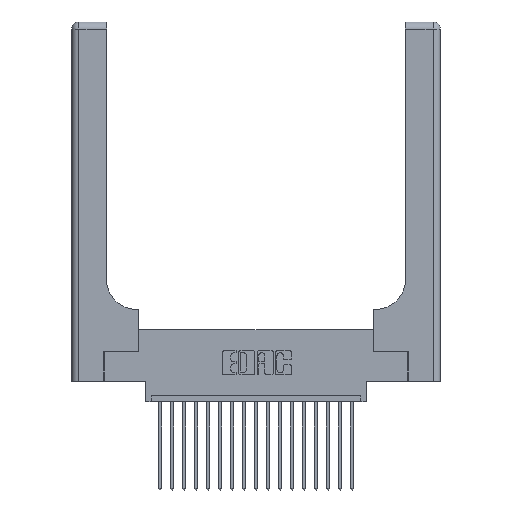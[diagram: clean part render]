
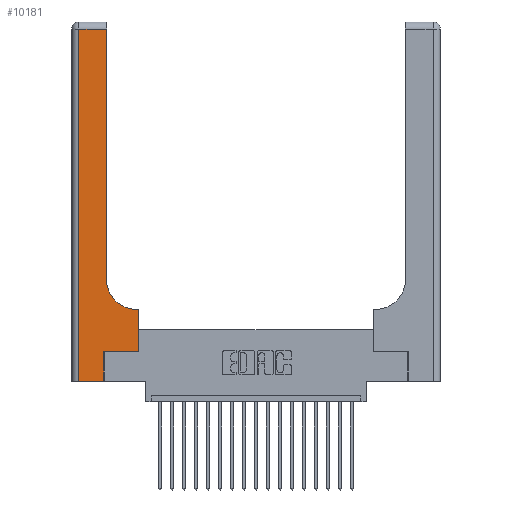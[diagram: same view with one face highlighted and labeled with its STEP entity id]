
A CAD part, top view. The second image highlights one B-rep face of the part: STEP entity #10181.
In plain terms, the highlighted planar face has unit normal (0, 0, 1).
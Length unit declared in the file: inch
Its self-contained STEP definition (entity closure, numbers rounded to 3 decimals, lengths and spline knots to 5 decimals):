
#115 = EDGE_CURVE ( 'NONE', #12358, #16170, #7274, .T. ) ;
#128 = CIRCLE ( 'NONE', #13776, 0.25 ) ;
#336 = ORIENTED_EDGE ( 'NONE', *, *, #13249, .T. ) ;
#466 = DIRECTION ( 'NONE',  ( -1., 0., 0. ) ) ;
#657 = ORIENTED_EDGE ( 'NONE', *, *, #16451, .T. ) ;
#726 = CARTESIAN_POINT ( 'NONE',  ( 0., 2.94, 0.37 ) ) ;
#1083 = CARTESIAN_POINT ( 'NONE',  ( 0.5585, 0.6, 0.37 ) ) ;
#1339 = VECTOR ( 'NONE', #5027, 39.37008 ) ;
#1526 = VERTEX_POINT ( 'NONE', #1083 ) ;
#1800 = VERTEX_POINT ( 'NONE', #20786 ) ;
#1990 = LINE ( 'NONE', #4769, #4318 ) ;
#2366 = DIRECTION ( 'NONE',  ( -1., 0., 0. ) ) ;
#2851 = ORIENTED_EDGE ( 'NONE', *, *, #115, .T. ) ;
#2908 = LINE ( 'NONE', #726, #19296 ) ;
#3039 = CARTESIAN_POINT ( 'NONE',  ( 0.2915, 3., 0.37 ) ) ;
#3593 = EDGE_CURVE ( 'NONE', #18591, #9116, #13647, .T. ) ;
#3760 = EDGE_CURVE ( 'NONE', #1800, #12052, #10984, .T. ) ;
#4318 = VECTOR ( 'NONE', #21324, 39.37008 ) ;
#4769 = CARTESIAN_POINT ( 'NONE',  ( 0.5585, 0.25, 0.37 ) ) ;
#4877 = CARTESIAN_POINT ( 'NONE',  ( 0.269, 0., 0.37 ) ) ;
#5027 = DIRECTION ( 'NONE',  ( 0., 1., 0. ) ) ;
#5097 = EDGE_CURVE ( 'NONE', #13422, #18591, #128, .T. ) ;
#5356 = VECTOR ( 'NONE', #19885, 39.37008 ) ;
#5435 = CARTESIAN_POINT ( 'NONE',  ( 0.269, 0.25, 0.37 ) ) ;
#5664 = DIRECTION ( 'NONE',  ( -1., 0., 0. ) ) ;
#6157 = CARTESIAN_POINT ( 'NONE',  ( 0.269, 0., 0.37 ) ) ;
#6214 = FACE_OUTER_BOUND ( 'NONE', #17953, .T. ) ;
#6238 = VECTOR ( 'NONE', #6935, 39.37008 ) ;
#6370 = DIRECTION ( 'NONE',  ( 0., 0., -1. ) ) ;
#6437 = VECTOR ( 'NONE', #19511, 39.37008 ) ;
#6935 = DIRECTION ( 'NONE',  ( 1., 0., 0. ) ) ;
#7274 = LINE ( 'NONE', #5435, #6238 ) ;
#7330 = ORIENTED_EDGE ( 'NONE', *, *, #13846, .T. ) ;
#7366 = CARTESIAN_POINT ( 'NONE',  ( 0.5415, 0.6, 0.37 ) ) ;
#7456 = AXIS2_PLACEMENT_3D ( 'NONE', #8731, #13614, #466 ) ;
#7781 = LINE ( 'NONE', #4877, #1339 ) ;
#8046 = CARTESIAN_POINT ( 'NONE',  ( 0.5585, 0.25, 0.37 ) ) ;
#8447 = ORIENTED_EDGE ( 'NONE', *, *, #5097, .T. ) ;
#8731 = CARTESIAN_POINT ( 'NONE',  ( 0., 3., 0.37 ) ) ;
#9116 = VERTEX_POINT ( 'NONE', #10461 ) ;
#10181 = ADVANCED_FACE ( 'NONE', ( #6214 ), #18722, .F. ) ;
#10461 = CARTESIAN_POINT ( 'NONE',  ( 0.2915, 2.94, 0.37 ) ) ;
#10879 = EDGE_CURVE ( 'NONE', #13463, #1800, #18939, .T. ) ;
#10984 = LINE ( 'NONE', #21500, #5356 ) ;
#11187 = DIRECTION ( 'NONE',  ( 0., 1., 0. ) ) ;
#11348 = DIRECTION ( 'NONE',  ( 1., 0., 0. ) ) ;
#11429 = CARTESIAN_POINT ( 'NONE',  ( 0.5415, 0.85, 0.37 ) ) ;
#12052 = VERTEX_POINT ( 'NONE', #6157 ) ;
#12358 = VERTEX_POINT ( 'NONE', #21292 ) ;
#13249 = EDGE_CURVE ( 'NONE', #1526, #13422, #17293, .T. ) ;
#13422 = VERTEX_POINT ( 'NONE', #7366 ) ;
#13463 = VERTEX_POINT ( 'NONE', #19082 ) ;
#13592 = ORIENTED_EDGE ( 'NONE', *, *, #3593, .T. ) ;
#13614 = DIRECTION ( 'NONE',  ( 0., 0., -1. ) ) ;
#13647 = LINE ( 'NONE', #3039, #17283 ) ;
#13776 = AXIS2_PLACEMENT_3D ( 'NONE', #11429, #6370, #11348 ) ;
#13846 = EDGE_CURVE ( 'NONE', #16170, #1526, #1990, .T. ) ;
#14249 = ORIENTED_EDGE ( 'NONE', *, *, #10879, .T. ) ;
#16170 = VERTEX_POINT ( 'NONE', #8046 ) ;
#16451 = EDGE_CURVE ( 'NONE', #9116, #13463, #2908, .T. ) ;
#16795 = ORIENTED_EDGE ( 'NONE', *, *, #3760, .T. ) ;
#17084 = CARTESIAN_POINT ( 'NONE',  ( 0.2915, 0.85, 0.37 ) ) ;
#17283 = VECTOR ( 'NONE', #11187, 39.37008 ) ;
#17293 = LINE ( 'NONE', #19020, #17811 ) ;
#17518 = EDGE_CURVE ( 'NONE', #12052, #12358, #7781, .T. ) ;
#17811 = VECTOR ( 'NONE', #5664, 39.37008 ) ;
#17953 = EDGE_LOOP ( 'NONE', ( #13592, #657, #14249, #16795, #19897, #2851, #7330, #336, #8447 ) ) ;
#18591 = VERTEX_POINT ( 'NONE', #17084 ) ;
#18722 = PLANE ( 'NONE',  #7456 ) ;
#18939 = LINE ( 'NONE', #20900, #6437 ) ;
#19020 = CARTESIAN_POINT ( 'NONE',  ( 0.2915, 0.6, 0.37 ) ) ;
#19082 = CARTESIAN_POINT ( 'NONE',  ( 0.06, 2.94, 0.37 ) ) ;
#19296 = VECTOR ( 'NONE', #2366, 39.37008 ) ;
#19511 = DIRECTION ( 'NONE',  ( 0., -1., 0. ) ) ;
#19885 = DIRECTION ( 'NONE',  ( 1., 0., 0. ) ) ;
#19897 = ORIENTED_EDGE ( 'NONE', *, *, #17518, .T. ) ;
#20786 = CARTESIAN_POINT ( 'NONE',  ( 0.06, 0., 0.37 ) ) ;
#20900 = CARTESIAN_POINT ( 'NONE',  ( 0.06, 3., 0.37 ) ) ;
#21292 = CARTESIAN_POINT ( 'NONE',  ( 0.269, 0.25, 0.37 ) ) ;
#21324 = DIRECTION ( 'NONE',  ( 0., 1., 0. ) ) ;
#21500 = CARTESIAN_POINT ( 'NONE',  ( 0., 0., 0.37 ) ) ;
